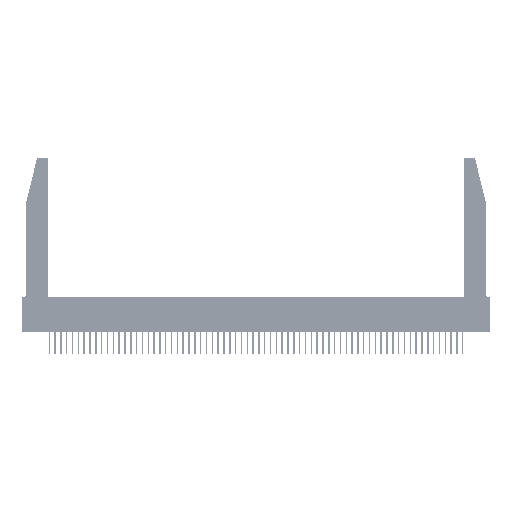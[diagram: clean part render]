
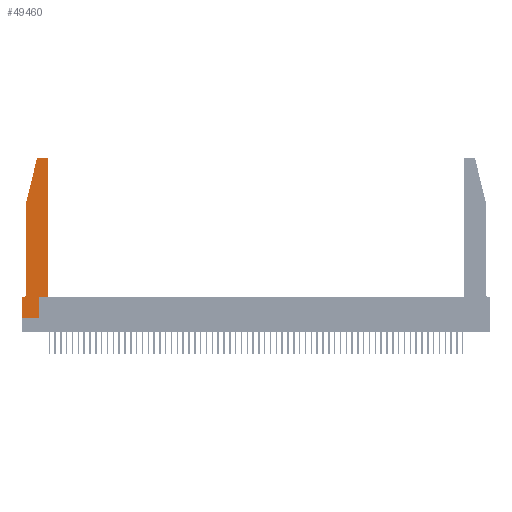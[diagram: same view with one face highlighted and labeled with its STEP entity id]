
A CAD part, top view. The second image highlights one B-rep face of the part: STEP entity #49460.
In plain terms, the highlighted planar face has unit normal (0, 0, 1).
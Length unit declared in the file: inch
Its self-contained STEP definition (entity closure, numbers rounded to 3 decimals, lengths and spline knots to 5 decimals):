
#116 = DIRECTION ( 'NONE',  ( -1., 0., 0. ) ) ;
#120 = ORIENTED_EDGE ( 'NONE', *, *, #4753, .T. ) ;
#347 = CARTESIAN_POINT ( 'NONE',  ( 0.0755, 0.35, 0.37 ) ) ;
#756 = DIRECTION ( 'NONE',  ( 1., 0., 0. ) ) ;
#772 = VECTOR ( 'NONE', #4218, 39.37008 ) ;
#1544 = DIRECTION ( 'NONE',  ( 0., -1., 0. ) ) ;
#2327 = DIRECTION ( 'NONE',  ( 0., 1., 0. ) ) ;
#2465 = EDGE_CURVE ( 'NONE', #18183, #31207, #36907, .T. ) ;
#2687 = ORIENTED_EDGE ( 'NONE', *, *, #28123, .T. ) ;
#3642 = VERTEX_POINT ( 'NONE', #20984 ) ;
#3924 = EDGE_LOOP ( 'NONE', ( #10457, #28579, #13009, #19483, #4412, #9123, #17256, #34046, #120, #19886, #2687, #43855 ) ) ;
#4049 = CARTESIAN_POINT ( 'NONE',  ( 0.0755, 2., 0.37 ) ) ;
#4218 = DIRECTION ( 'NONE',  ( 0., 1., 0. ) ) ;
#4412 = ORIENTED_EDGE ( 'NONE', *, *, #46009, .T. ) ;
#4441 = PLANE ( 'NONE',  #22929 ) ;
#4460 = VERTEX_POINT ( 'NONE', #23779 ) ;
#4625 = CARTESIAN_POINT ( 'NONE',  ( 0., 0.35, 0.37 ) ) ;
#4753 = EDGE_CURVE ( 'NONE', #41356, #18183, #29108, .T. ) ;
#4811 = EDGE_CURVE ( 'NONE', #38609, #39697, #22877, .T. ) ;
#4828 = DIRECTION ( 'NONE',  ( 1., 0., 0. ) ) ;
#5081 = CARTESIAN_POINT ( 'NONE',  ( 0., 0.35, 0.37 ) ) ;
#6857 = DIRECTION ( 'NONE',  ( -0.239, -0.971, 0. ) ) ;
#7058 = LINE ( 'NONE', #19787, #11931 ) ;
#8128 = CARTESIAN_POINT ( 'NONE',  ( 0.0755, 2., 0.37 ) ) ;
#9123 = ORIENTED_EDGE ( 'NONE', *, *, #40538, .T. ) ;
#10457 = ORIENTED_EDGE ( 'NONE', *, *, #39093, .T. ) ;
#10886 = CARTESIAN_POINT ( 'NONE',  ( 0.2865, 0.35, 0.37 ) ) ;
#11050 = DIRECTION ( 'NONE',  ( 1., 0., 0. ) ) ;
#11931 = VECTOR ( 'NONE', #6857, 39.37008 ) ;
#12394 = CARTESIAN_POINT ( 'NONE',  ( 0., 0., 0.37 ) ) ;
#13009 = ORIENTED_EDGE ( 'NONE', *, *, #39605, .T. ) ;
#13695 = DIRECTION ( 'NONE',  ( 0., 0., 1. ) ) ;
#15187 = CARTESIAN_POINT ( 'NONE',  ( 0.284, 2.75, 0.37 ) ) ;
#15797 = FACE_OUTER_BOUND ( 'NONE', #3924, .T. ) ;
#16636 = VERTEX_POINT ( 'NONE', #12394 ) ;
#17256 = ORIENTED_EDGE ( 'NONE', *, *, #33880, .T. ) ;
#18046 = CARTESIAN_POINT ( 'NONE',  ( 0.4505, 0.35, 0.37 ) ) ;
#18183 = VERTEX_POINT ( 'NONE', #10886 ) ;
#19483 = ORIENTED_EDGE ( 'NONE', *, *, #4811, .T. ) ;
#19523 = DIRECTION ( 'NONE',  ( 0., 0., 1. ) ) ;
#19592 = CARTESIAN_POINT ( 'NONE',  ( 0.2865, 0., 0.37 ) ) ;
#19787 = CARTESIAN_POINT ( 'NONE',  ( 0.0755, 2., 0.37 ) ) ;
#19886 = ORIENTED_EDGE ( 'NONE', *, *, #2465, .T. ) ;
#20984 = CARTESIAN_POINT ( 'NONE',  ( 0.25487, 2.72718, 0.37 ) ) ;
#21240 = VERTEX_POINT ( 'NONE', #5081 ) ;
#22877 = LINE ( 'NONE', #8128, #55432 ) ;
#22929 = AXIS2_PLACEMENT_3D ( 'NONE', #4625, #43935, #4828 ) ;
#23779 = CARTESIAN_POINT ( 'NONE',  ( 0.0055, 0.35, 0.37 ) ) ;
#24014 = CIRCLE ( 'NONE', #32336, 0.03 ) ;
#24721 = CARTESIAN_POINT ( 'NONE',  ( 0., 0., 0.37 ) ) ;
#26077 = CARTESIAN_POINT ( 'NONE',  ( 0.2865, 0.35, 0.37 ) ) ;
#26332 = VECTOR ( 'NONE', #42351, 39.37008 ) ;
#26534 = DIRECTION ( 'NONE',  ( 1., 0., 0. ) ) ;
#26559 = CARTESIAN_POINT ( 'NONE',  ( 0.0055, 0.42, 0.37 ) ) ;
#27144 = AXIS2_PLACEMENT_3D ( 'NONE', #51086, #19523, #11050 ) ;
#27207 = CARTESIAN_POINT ( 'NONE',  ( 0.4205, 2.72, 0.37 ) ) ;
#27559 = DIRECTION ( 'NONE',  ( -1., 0., 0. ) ) ;
#27636 = CARTESIAN_POINT ( 'NONE',  ( 0., 0., 0.37 ) ) ;
#28123 = EDGE_CURVE ( 'NONE', #31207, #54332, #50594, .T. ) ;
#28423 = VECTOR ( 'NONE', #2327, 39.37008 ) ;
#28579 = ORIENTED_EDGE ( 'NONE', *, *, #41881, .T. ) ;
#29108 = LINE ( 'NONE', #26077, #772 ) ;
#29704 = LINE ( 'NONE', #27636, #40810 ) ;
#30292 = CIRCLE ( 'NONE', #27144, 0.03 ) ;
#31207 = VERTEX_POINT ( 'NONE', #55504 ) ;
#32336 = AXIS2_PLACEMENT_3D ( 'NONE', #27207, #13695, #756 ) ;
#33795 = CARTESIAN_POINT ( 'NONE',  ( 0.4505, 2.72, 0.37 ) ) ;
#33880 = EDGE_CURVE ( 'NONE', #21240, #16636, #29704, .T. ) ;
#34046 = ORIENTED_EDGE ( 'NONE', *, *, #50637, .T. ) ;
#34324 = CARTESIAN_POINT ( 'NONE',  ( 0.4205, 2.75, 0.37 ) ) ;
#35491 = CIRCLE ( 'NONE', #49897, 0.07 ) ;
#36771 = VECTOR ( 'NONE', #38652, 39.37008 ) ;
#36907 = LINE ( 'NONE', #18046, #37646 ) ;
#37634 = VERTEX_POINT ( 'NONE', #15187 ) ;
#37646 = VECTOR ( 'NONE', #26534, 39.37008 ) ;
#38609 = VERTEX_POINT ( 'NONE', #4049 ) ;
#38652 = DIRECTION ( 'NONE',  ( -1., 0., 0. ) ) ;
#39093 = EDGE_CURVE ( 'NONE', #46856, #37634, #54772, .T. ) ;
#39605 = EDGE_CURVE ( 'NONE', #3642, #38609, #7058, .T. ) ;
#39697 = VERTEX_POINT ( 'NONE', #42648 ) ;
#40538 = EDGE_CURVE ( 'NONE', #4460, #21240, #47772, .T. ) ;
#40810 = VECTOR ( 'NONE', #1544, 39.37008 ) ;
#41356 = VERTEX_POINT ( 'NONE', #19592 ) ;
#41881 = EDGE_CURVE ( 'NONE', #37634, #3642, #30292, .T. ) ;
#42351 = DIRECTION ( 'NONE',  ( 1., 0., 0. ) ) ;
#42374 = EDGE_CURVE ( 'NONE', #54332, #46856, #24014, .T. ) ;
#42648 = CARTESIAN_POINT ( 'NONE',  ( 0.0755, 0.42, 0.37 ) ) ;
#43090 = CARTESIAN_POINT ( 'NONE',  ( 0.2605, 2.75, 0.37 ) ) ;
#43521 = DIRECTION ( 'NONE',  ( 0., -1., 0. ) ) ;
#43855 = ORIENTED_EDGE ( 'NONE', *, *, #42374, .T. ) ;
#43935 = DIRECTION ( 'NONE',  ( 0., 0., 1. ) ) ;
#44388 = DIRECTION ( 'NONE',  ( 0., 0., -1. ) ) ;
#46009 = EDGE_CURVE ( 'NONE', #39697, #4460, #35491, .T. ) ;
#46856 = VERTEX_POINT ( 'NONE', #34324 ) ;
#47772 = LINE ( 'NONE', #347, #49837 ) ;
#49460 = ADVANCED_FACE ( 'NONE', ( #15797 ), #4441, .T. ) ;
#49837 = VECTOR ( 'NONE', #27559, 39.37008 ) ;
#49897 = AXIS2_PLACEMENT_3D ( 'NONE', #26559, #44388, #116 ) ;
#50594 = LINE ( 'NONE', #50890, #28423 ) ;
#50637 = EDGE_CURVE ( 'NONE', #16636, #41356, #55441, .T. ) ;
#50890 = CARTESIAN_POINT ( 'NONE',  ( 0.4505, 0.35, 0.37 ) ) ;
#51086 = CARTESIAN_POINT ( 'NONE',  ( 0.284, 2.72, 0.37 ) ) ;
#54332 = VERTEX_POINT ( 'NONE', #33795 ) ;
#54772 = LINE ( 'NONE', #43090, #36771 ) ;
#55432 = VECTOR ( 'NONE', #43521, 39.37008 ) ;
#55441 = LINE ( 'NONE', #24721, #26332 ) ;
#55504 = CARTESIAN_POINT ( 'NONE',  ( 0.4505, 0.35, 0.37 ) ) ;
